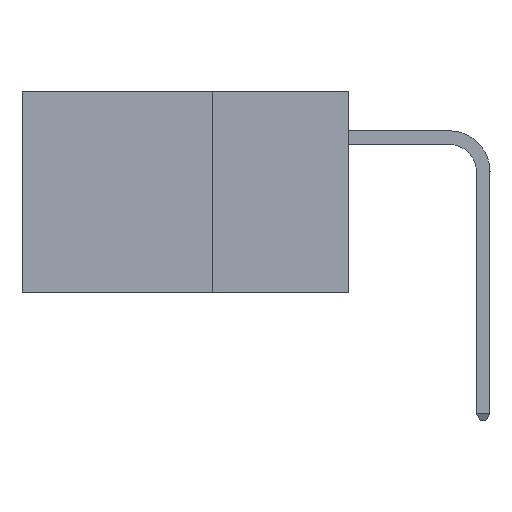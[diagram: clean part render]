
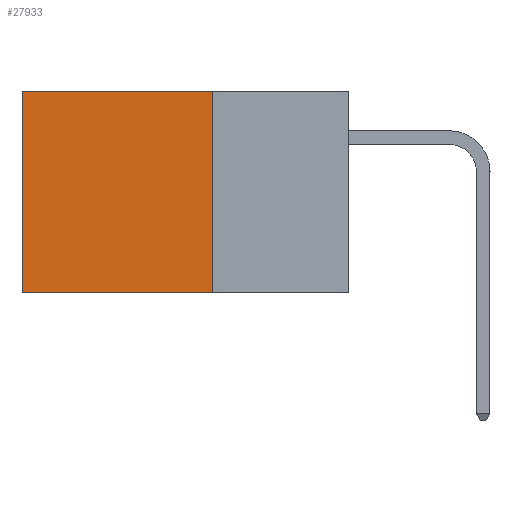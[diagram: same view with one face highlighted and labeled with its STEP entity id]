
A CAD part, left-side view. The second image highlights one B-rep face of the part: STEP entity #27933.
In plain terms, the highlighted planar face has unit normal (-1, 0, 0).
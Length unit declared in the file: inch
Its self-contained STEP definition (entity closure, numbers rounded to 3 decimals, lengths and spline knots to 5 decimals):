
#255 = CARTESIAN_POINT ( 'NONE',  ( 0.2875, 0.25, 0. ) ) ;
#370 = DIRECTION ( 'NONE',  ( 1., 0., 0. ) ) ;
#1428 = EDGE_CURVE ( 'NONE', #7887, #2562, #2472, .T. ) ;
#1481 = CARTESIAN_POINT ( 'NONE',  ( 0.2875, 0.25, 0. ) ) ;
#2117 = VERTEX_POINT ( 'NONE', #9604 ) ;
#2300 = DIRECTION ( 'NONE',  ( 0., 1., 0. ) ) ;
#2472 = LINE ( 'NONE', #1481, #25515 ) ;
#2562 = VERTEX_POINT ( 'NONE', #19769 ) ;
#3912 = EDGE_CURVE ( 'NONE', #2562, #2117, #25710, .T. ) ;
#4172 = VECTOR ( 'NONE', #8189, 39.37008 ) ;
#5629 = AXIS2_PLACEMENT_3D ( 'NONE', #255, #370, #17840 ) ;
#5642 = CARTESIAN_POINT ( 'NONE',  ( 0.2875, 0.25, 0. ) ) ;
#5644 = LINE ( 'NONE', #11021, #17320 ) ;
#6009 = VERTEX_POINT ( 'NONE', #25040 ) ;
#7887 = VERTEX_POINT ( 'NONE', #25154 ) ;
#8189 = DIRECTION ( 'NONE',  ( 0., 0., -1. ) ) ;
#9604 = CARTESIAN_POINT ( 'NONE',  ( 0.2875, 0.6, -0.37 ) ) ;
#10405 = PLANE ( 'NONE',  #5629 ) ;
#10581 = DIRECTION ( 'NONE',  ( 0., 0., -1. ) ) ;
#11021 = CARTESIAN_POINT ( 'NONE',  ( 0.2875, 0.25, -0.37 ) ) ;
#13116 = EDGE_LOOP ( 'NONE', ( #15723, #15041, #23841, #31144 ) ) ;
#13550 = VECTOR ( 'NONE', #10581, 39.37008 ) ;
#15041 = ORIENTED_EDGE ( 'NONE', *, *, #22203, .F. ) ;
#15723 = ORIENTED_EDGE ( 'NONE', *, *, #3912, .T. ) ;
#17320 = VECTOR ( 'NONE', #30326, 39.37008 ) ;
#17840 = DIRECTION ( 'NONE',  ( 0., 0., -1. ) ) ;
#19769 = CARTESIAN_POINT ( 'NONE',  ( 0.2875, 0.6, 0. ) ) ;
#22203 = EDGE_CURVE ( 'NONE', #6009, #2117, #5644, .T. ) ;
#23841 = ORIENTED_EDGE ( 'NONE', *, *, #29545, .F. ) ;
#25040 = CARTESIAN_POINT ( 'NONE',  ( 0.2875, 0.25, -0.37 ) ) ;
#25154 = CARTESIAN_POINT ( 'NONE',  ( 0.2875, 0.25, 0. ) ) ;
#25194 = CARTESIAN_POINT ( 'NONE',  ( 0.2875, 0.6, 0. ) ) ;
#25515 = VECTOR ( 'NONE', #2300, 39.37008 ) ;
#25710 = LINE ( 'NONE', #25194, #13550 ) ;
#27933 = ADVANCED_FACE ( 'NONE', ( #28068 ), #10405, .F. ) ;
#28068 = FACE_OUTER_BOUND ( 'NONE', #13116, .T. ) ;
#29545 = EDGE_CURVE ( 'NONE', #7887, #6009, #30147, .T. ) ;
#30147 = LINE ( 'NONE', #5642, #4172 ) ;
#30326 = DIRECTION ( 'NONE',  ( 0., 1., 0. ) ) ;
#31144 = ORIENTED_EDGE ( 'NONE', *, *, #1428, .T. ) ;
